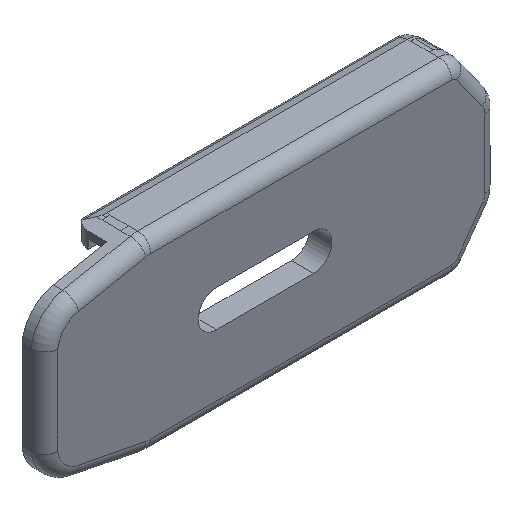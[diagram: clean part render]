
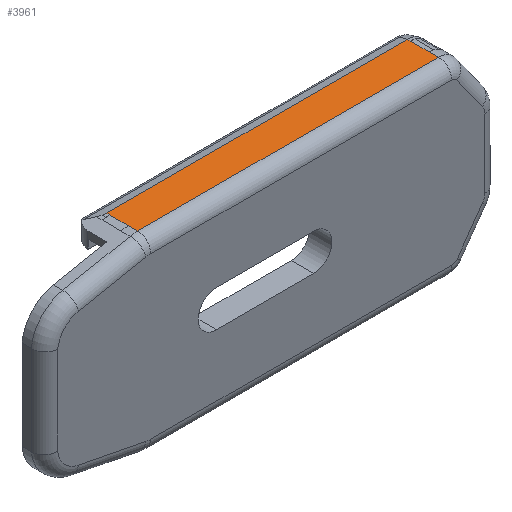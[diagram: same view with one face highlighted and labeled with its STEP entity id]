
A CAD part, isometric view. The second image highlights one B-rep face of the part: STEP entity #3961.
In plain terms, the highlighted face is planar.
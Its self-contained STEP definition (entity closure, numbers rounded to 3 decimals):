
#31 = VERTEX_POINT ( 'NONE', #2997 ) ;
#150 = VECTOR ( 'NONE', #941, 1000. ) ;
#198 = CARTESIAN_POINT ( 'NONE',  ( 14.2, 4.36, 52.748 ) ) ;
#472 = LINE ( 'NONE', #2635, #1578 ) ;
#497 = DIRECTION ( 'NONE',  ( 0., -1., 0. ) ) ;
#552 = LINE ( 'NONE', #198, #2452 ) ;
#619 = VERTEX_POINT ( 'NONE', #2463 ) ;
#653 = LINE ( 'NONE', #3069, #3334 ) ;
#737 = EDGE_LOOP ( 'NONE', ( #3855, #1114, #1842, #3654, #1371, #4368, #4017, #901 ) ) ;
#750 = VERTEX_POINT ( 'NONE', #2054 ) ;
#824 = LINE ( 'NONE', #3002, #3047 ) ;
#882 = VECTOR ( 'NONE', #3096, 1000. ) ;
#901 = ORIENTED_EDGE ( 'NONE', *, *, #3690, .F. ) ;
#941 = DIRECTION ( 'NONE',  ( 0., -1., 0. ) ) ;
#975 = CARTESIAN_POINT ( 'NONE',  ( 14.2, -0.94, 7. ) ) ;
#1060 = DIRECTION ( 'NONE',  ( 0., -1., 0. ) ) ;
#1068 = LINE ( 'NONE', #3502, #882 ) ;
#1114 = ORIENTED_EDGE ( 'NONE', *, *, #3823, .T. ) ;
#1123 = AXIS2_PLACEMENT_3D ( 'NONE', #1990, #2674, #4055 ) ;
#1204 = LINE ( 'NONE', #1618, #4523 ) ;
#1237 = PLANE ( 'NONE',  #1123 ) ;
#1254 = LINE ( 'NONE', #3432, #150 ) ;
#1371 = ORIENTED_EDGE ( 'NONE', *, *, #4587, .T. ) ;
#1452 = EDGE_CURVE ( 'NONE', #3359, #750, #824, .T. ) ;
#1478 = EDGE_CURVE ( 'NONE', #2648, #619, #472, .T. ) ;
#1578 = VECTOR ( 'NONE', #3022, 1000. ) ;
#1618 = CARTESIAN_POINT ( 'NONE',  ( 14.2, -0.94, 52.748 ) ) ;
#1782 = CARTESIAN_POINT ( 'NONE',  ( 14.2, 1.91, 7. ) ) ;
#1842 = ORIENTED_EDGE ( 'NONE', *, *, #3608, .T. ) ;
#1990 = CARTESIAN_POINT ( 'NONE',  ( 14.2, -0.94, 52.748 ) ) ;
#2033 = DIRECTION ( 'NONE',  ( 0., -1., 0. ) ) ;
#2054 = CARTESIAN_POINT ( 'NONE',  ( 14.2, -2.36, 7. ) ) ;
#2081 = CARTESIAN_POINT ( 'NONE',  ( 14.2, 2.36, 52.748 ) ) ;
#2348 = CARTESIAN_POINT ( 'NONE',  ( 14.2, -2.36, 52.748 ) ) ;
#2379 = VECTOR ( 'NONE', #3915, 1000. ) ;
#2452 = VECTOR ( 'NONE', #2033, 1000. ) ;
#2463 = CARTESIAN_POINT ( 'NONE',  ( 14.2, -0.94, 52.748 ) ) ;
#2555 = EDGE_CURVE ( 'NONE', #4132, #3819, #1068, .T. ) ;
#2635 = CARTESIAN_POINT ( 'NONE',  ( 14.2, 1.91, 52.748 ) ) ;
#2648 = VERTEX_POINT ( 'NONE', #3240 ) ;
#2674 = DIRECTION ( 'NONE',  ( -1., 0., 0. ) ) ;
#2709 = CARTESIAN_POINT ( 'NONE',  ( 14.2, 2.36, 7. ) ) ;
#2978 = EDGE_CURVE ( 'NONE', #3345, #750, #653, .T. ) ;
#2997 = CARTESIAN_POINT ( 'NONE',  ( 14.2, 2.36, 52.748 ) ) ;
#3002 = CARTESIAN_POINT ( 'NONE',  ( 14.2, -2.36, 7. ) ) ;
#3022 = DIRECTION ( 'NONE',  ( 0., -1., 0. ) ) ;
#3047 = VECTOR ( 'NONE', #4411, 1000. ) ;
#3069 = CARTESIAN_POINT ( 'NONE',  ( 14.2, -0.94, 7. ) ) ;
#3096 = DIRECTION ( 'NONE',  ( 0., -1., 0. ) ) ;
#3240 = CARTESIAN_POINT ( 'NONE',  ( 14.2, 1.91, 52.748 ) ) ;
#3334 = VECTOR ( 'NONE', #1060, 1000. ) ;
#3345 = VERTEX_POINT ( 'NONE', #975 ) ;
#3359 = VERTEX_POINT ( 'NONE', #2348 ) ;
#3432 = CARTESIAN_POINT ( 'NONE',  ( 14.2, 1.91, 7. ) ) ;
#3502 = CARTESIAN_POINT ( 'NONE',  ( 14.2, 4.36, 7. ) ) ;
#3608 = EDGE_CURVE ( 'NONE', #31, #2648, #552, .T. ) ;
#3654 = ORIENTED_EDGE ( 'NONE', *, *, #1478, .T. ) ;
#3690 = EDGE_CURVE ( 'NONE', #3819, #3345, #1254, .T. ) ;
#3784 = FACE_OUTER_BOUND ( 'NONE', #737, .T. ) ;
#3819 = VERTEX_POINT ( 'NONE', #1782 ) ;
#3823 = EDGE_CURVE ( 'NONE', #4132, #31, #4163, .T. ) ;
#3855 = ORIENTED_EDGE ( 'NONE', *, *, #2555, .F. ) ;
#3915 = DIRECTION ( 'NONE',  ( 0., 0., 1. ) ) ;
#3961 = ADVANCED_FACE ( 'NONE', ( #3784 ), #1237, .F. ) ;
#4017 = ORIENTED_EDGE ( 'NONE', *, *, #2978, .F. ) ;
#4055 = DIRECTION ( 'NONE',  ( 0., 0., 1. ) ) ;
#4132 = VERTEX_POINT ( 'NONE', #2709 ) ;
#4163 = LINE ( 'NONE', #2081, #2379 ) ;
#4368 = ORIENTED_EDGE ( 'NONE', *, *, #1452, .T. ) ;
#4411 = DIRECTION ( 'NONE',  ( 0., 0., -1. ) ) ;
#4523 = VECTOR ( 'NONE', #497, 1000. ) ;
#4587 = EDGE_CURVE ( 'NONE', #619, #3359, #1204, .T. ) ;
